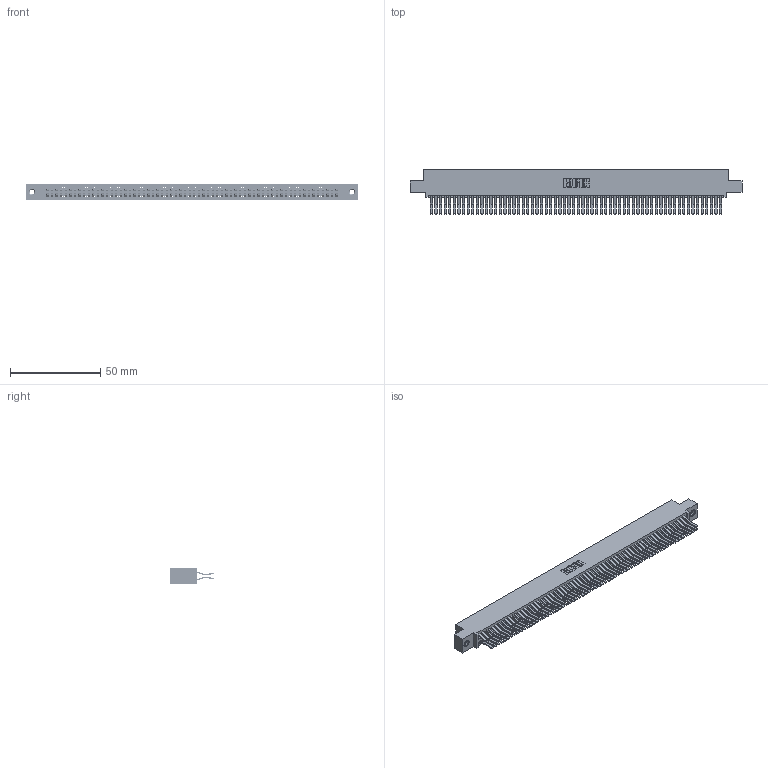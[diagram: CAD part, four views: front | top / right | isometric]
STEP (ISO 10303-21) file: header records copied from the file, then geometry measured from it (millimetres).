
FILE_DESCRIPTION (( 'STEP AP203' ), '1' );
FILE_NAME ('345-128-560-507.STEP', '2018-10-19T22:25:12', ( '' ), ( '' ), 'SwSTEP 2.0', 'SolidWorks 2016', '' );
FILE_SCHEMA (( 'CONFIG_CONTROL_DESIGN' ));
Length unit declared in the file: inch
Products named in the file (4): 345-128-560-507; 345-292-001_560 Tail; 345 Part_0.110 Offset - 0.156 Dia-TI; 345-250-001_345-250-005-103
Assembly tree (131 placements, depth 2):
  345-128-560-507
    345 Part_0.110 Offset - 0.156 Dia-TI
    345-292-001_560 Tail  x128
    345-250-001_345-250-005-103  x2
Bounding box: 183.77 x 24.45 x 9.4 mm (x, y, z)
Volume: 18807.8 mm3; surface area: 30505.7 mm2
Topology: 131 solids, 131 shells, 6846 faces, 20329 edges, 13374 vertices
Faces by surface type: plane 4340, cylinder 2490, cone 12, torus 4
Entity records: 48660 total; most frequent: CARTESIAN_POINT 8119, ORIENTED_EDGE 8046, DIRECTION 7161, EDGE_CURVE 4023, VECTOR 3611, LINE 3611, VERTEX_POINT 2676, AXIS2_PLACEMENT_3D 1775
